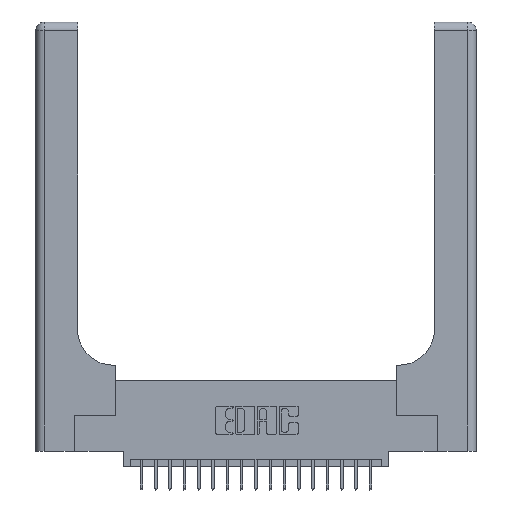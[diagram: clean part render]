
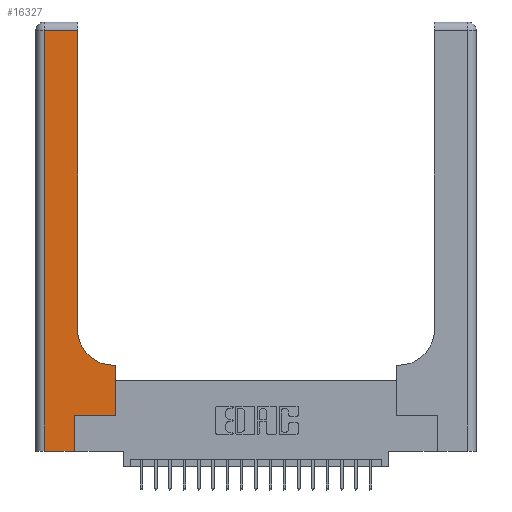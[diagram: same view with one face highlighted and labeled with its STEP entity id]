
A CAD part, top view. The second image highlights one B-rep face of the part: STEP entity #16327.
In plain terms, the highlighted planar face has unit normal (0, 0, 1).
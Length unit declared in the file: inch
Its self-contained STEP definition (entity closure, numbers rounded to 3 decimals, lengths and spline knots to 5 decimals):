
#22 = EDGE_CURVE ( 'NONE', #4698, #5597, #5431, .T. ) ;
#46 = VERTEX_POINT ( 'NONE', #10252 ) ;
#825 = LINE ( 'NONE', #8427, #18471 ) ;
#839 = VERTEX_POINT ( 'NONE', #19274 ) ;
#1159 = ORIENTED_EDGE ( 'NONE', *, *, #8653, .T. ) ;
#1626 = DIRECTION ( 'NONE',  ( 1., 0., 0. ) ) ;
#1841 = VERTEX_POINT ( 'NONE', #12335 ) ;
#1915 = LINE ( 'NONE', #21245, #15563 ) ;
#2386 = EDGE_CURVE ( 'NONE', #12198, #6201, #10977, .T. ) ;
#2416 = CARTESIAN_POINT ( 'NONE',  ( 0.5415, 0.85, 0.37 ) ) ;
#2439 = EDGE_LOOP ( 'NONE', ( #13149, #9391, #10551, #1159, #7667, #5088, #15671, #17671, #12709 ) ) ;
#2522 = DIRECTION ( 'NONE',  ( 1., 0., 0. ) ) ;
#2579 = DIRECTION ( 'NONE',  ( 0., 1., 0. ) ) ;
#2616 = CARTESIAN_POINT ( 'NONE',  ( 0.269, 0.25, 0.37 ) ) ;
#2950 = AXIS2_PLACEMENT_3D ( 'NONE', #8899, #8451, #3368 ) ;
#3099 = DIRECTION ( 'NONE',  ( 0., 1., 0. ) ) ;
#3231 = PLANE ( 'NONE',  #2950 ) ;
#3234 = EDGE_CURVE ( 'NONE', #17950, #839, #8551, .T. ) ;
#3368 = DIRECTION ( 'NONE',  ( -1., 0., 0. ) ) ;
#3633 = CARTESIAN_POINT ( 'NONE',  ( 0.2915, 3., 0.37 ) ) ;
#4157 = DIRECTION ( 'NONE',  ( 1., 0., 0. ) ) ;
#4698 = VERTEX_POINT ( 'NONE', #19002 ) ;
#4894 = CARTESIAN_POINT ( 'NONE',  ( 0.269, 0., 0.37 ) ) ;
#4903 = VECTOR ( 'NONE', #10357, 39.37008 ) ;
#5088 = ORIENTED_EDGE ( 'NONE', *, *, #2386, .T. ) ;
#5431 = CIRCLE ( 'NONE', #16679, 0.25 ) ;
#5597 = VERTEX_POINT ( 'NONE', #19824 ) ;
#6046 = VECTOR ( 'NONE', #16247, 39.37008 ) ;
#6201 = VERTEX_POINT ( 'NONE', #21568 ) ;
#6207 = EDGE_CURVE ( 'NONE', #14882, #4698, #6593, .T. ) ;
#6476 = VECTOR ( 'NONE', #2522, 39.37008 ) ;
#6538 = FACE_OUTER_BOUND ( 'NONE', #2439, .T. ) ;
#6593 = LINE ( 'NONE', #16477, #6046 ) ;
#7667 = ORIENTED_EDGE ( 'NONE', *, *, #12739, .T. ) ;
#8427 = CARTESIAN_POINT ( 'NONE',  ( 0., 0., 0.37 ) ) ;
#8451 = DIRECTION ( 'NONE',  ( 0., 0., -1. ) ) ;
#8551 = LINE ( 'NONE', #19611, #21618 ) ;
#8653 = EDGE_CURVE ( 'NONE', #839, #46, #825, .T. ) ;
#8657 = EDGE_CURVE ( 'NONE', #1841, #17950, #13629, .T. ) ;
#8899 = CARTESIAN_POINT ( 'NONE',  ( 0., 3., 0.37 ) ) ;
#9391 = ORIENTED_EDGE ( 'NONE', *, *, #8657, .T. ) ;
#9446 = LINE ( 'NONE', #3633, #4903 ) ;
#10252 = CARTESIAN_POINT ( 'NONE',  ( 0.269, 0., 0.37 ) ) ;
#10357 = DIRECTION ( 'NONE',  ( 0., 1., 0. ) ) ;
#10551 = ORIENTED_EDGE ( 'NONE', *, *, #3234, .T. ) ;
#10977 = LINE ( 'NONE', #17563, #6476 ) ;
#12198 = VERTEX_POINT ( 'NONE', #2616 ) ;
#12335 = CARTESIAN_POINT ( 'NONE',  ( 0.2915, 2.94, 0.37 ) ) ;
#12709 = ORIENTED_EDGE ( 'NONE', *, *, #22, .T. ) ;
#12739 = EDGE_CURVE ( 'NONE', #46, #12198, #18843, .T. ) ;
#13149 = ORIENTED_EDGE ( 'NONE', *, *, #16938, .T. ) ;
#13310 = CARTESIAN_POINT ( 'NONE',  ( 0.06, 2.94, 0.37 ) ) ;
#13629 = LINE ( 'NONE', #13717, #21365 ) ;
#13717 = CARTESIAN_POINT ( 'NONE',  ( 0., 2.94, 0.37 ) ) ;
#13856 = DIRECTION ( 'NONE',  ( -1., 0., 0. ) ) ;
#13912 = EDGE_CURVE ( 'NONE', #6201, #14882, #1915, .T. ) ;
#14381 = DIRECTION ( 'NONE',  ( 0., 0., -1. ) ) ;
#14882 = VERTEX_POINT ( 'NONE', #18902 ) ;
#15563 = VECTOR ( 'NONE', #2579, 39.37008 ) ;
#15671 = ORIENTED_EDGE ( 'NONE', *, *, #13912, .T. ) ;
#16247 = DIRECTION ( 'NONE',  ( -1., 0., 0. ) ) ;
#16327 = ADVANCED_FACE ( 'NONE', ( #6538 ), #3231, .F. ) ;
#16477 = CARTESIAN_POINT ( 'NONE',  ( 0.2915, 0.6, 0.37 ) ) ;
#16679 = AXIS2_PLACEMENT_3D ( 'NONE', #2416, #14381, #4157 ) ;
#16938 = EDGE_CURVE ( 'NONE', #5597, #1841, #9446, .T. ) ;
#17563 = CARTESIAN_POINT ( 'NONE',  ( 0.269, 0.25, 0.37 ) ) ;
#17671 = ORIENTED_EDGE ( 'NONE', *, *, #6207, .T. ) ;
#17950 = VERTEX_POINT ( 'NONE', #13310 ) ;
#18324 = VECTOR ( 'NONE', #3099, 39.37008 ) ;
#18471 = VECTOR ( 'NONE', #1626, 39.37008 ) ;
#18843 = LINE ( 'NONE', #4894, #18324 ) ;
#18902 = CARTESIAN_POINT ( 'NONE',  ( 0.5585, 0.6, 0.37 ) ) ;
#19002 = CARTESIAN_POINT ( 'NONE',  ( 0.5415, 0.6, 0.37 ) ) ;
#19274 = CARTESIAN_POINT ( 'NONE',  ( 0.06, 0., 0.37 ) ) ;
#19315 = DIRECTION ( 'NONE',  ( 0., -1., 0. ) ) ;
#19611 = CARTESIAN_POINT ( 'NONE',  ( 0.06, 3., 0.37 ) ) ;
#19824 = CARTESIAN_POINT ( 'NONE',  ( 0.2915, 0.85, 0.37 ) ) ;
#21245 = CARTESIAN_POINT ( 'NONE',  ( 0.5585, 0.25, 0.37 ) ) ;
#21365 = VECTOR ( 'NONE', #13856, 39.37008 ) ;
#21568 = CARTESIAN_POINT ( 'NONE',  ( 0.5585, 0.25, 0.37 ) ) ;
#21618 = VECTOR ( 'NONE', #19315, 39.37008 ) ;
